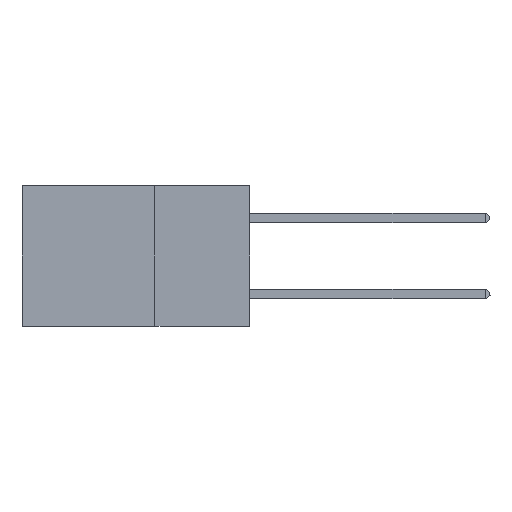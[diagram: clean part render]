
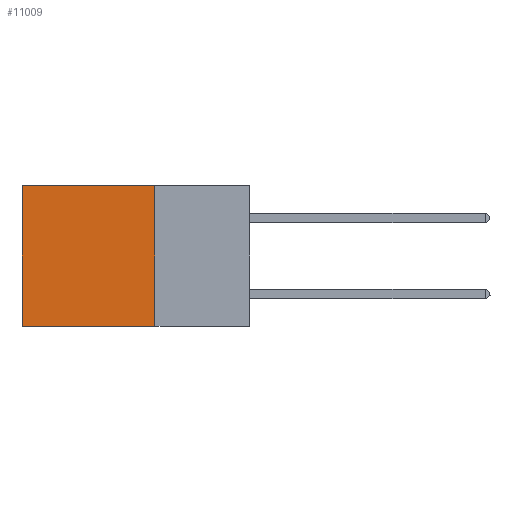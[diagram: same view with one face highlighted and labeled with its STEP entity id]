
A CAD part, left-side view. The second image highlights one B-rep face of the part: STEP entity #11009.
In plain terms, the highlighted planar face has unit normal (-1, 0, 0).
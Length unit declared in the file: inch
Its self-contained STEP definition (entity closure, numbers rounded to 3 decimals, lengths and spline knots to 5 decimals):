
#884 = DIRECTION ( 'NONE',  ( 0., 0., -1. ) ) ;
#1632 = VECTOR ( 'NONE', #884, 39.37008 ) ;
#2352 = CARTESIAN_POINT ( 'NONE',  ( 0.2875, 0.25, 0. ) ) ;
#2392 = ORIENTED_EDGE ( 'NONE', *, *, #11553, .T. ) ;
#2393 = CARTESIAN_POINT ( 'NONE',  ( 0.2875, 0.6, 0. ) ) ;
#2508 = PLANE ( 'NONE',  #12608 ) ;
#3537 = VERTEX_POINT ( 'NONE', #11201 ) ;
#4479 = ORIENTED_EDGE ( 'NONE', *, *, #10463, .F. ) ;
#6075 = EDGE_CURVE ( 'NONE', #9899, #13327, #8644, .T. ) ;
#6918 = DIRECTION ( 'NONE',  ( 0., 1., 0. ) ) ;
#7682 = DIRECTION ( 'NONE',  ( 0., 0., -1. ) ) ;
#7990 = CARTESIAN_POINT ( 'NONE',  ( 0.2875, 0.6, 0. ) ) ;
#8022 = VECTOR ( 'NONE', #6918, 39.37008 ) ;
#8190 = CARTESIAN_POINT ( 'NONE',  ( 0.2875, 0.25, 0. ) ) ;
#8644 = LINE ( 'NONE', #19015, #1632 ) ;
#9435 = LINE ( 'NONE', #2352, #8022 ) ;
#9899 = VERTEX_POINT ( 'NONE', #8190 ) ;
#10092 = DIRECTION ( 'NONE',  ( 0., 0., -1. ) ) ;
#10463 = EDGE_CURVE ( 'NONE', #13327, #3537, #11490, .T. ) ;
#10764 = LINE ( 'NONE', #7990, #15193 ) ;
#11009 = ADVANCED_FACE ( 'NONE', ( #17859 ), #2508, .F. ) ;
#11201 = CARTESIAN_POINT ( 'NONE',  ( 0.2875, 0.6, -0.37 ) ) ;
#11490 = LINE ( 'NONE', #17861, #13829 ) ;
#11553 = EDGE_CURVE ( 'NONE', #9899, #19079, #9435, .T. ) ;
#11558 = EDGE_LOOP ( 'NONE', ( #11972, #4479, #18314, #2392 ) ) ;
#11972 = ORIENTED_EDGE ( 'NONE', *, *, #12540, .T. ) ;
#12540 = EDGE_CURVE ( 'NONE', #19079, #3537, #10764, .T. ) ;
#12608 = AXIS2_PLACEMENT_3D ( 'NONE', #17445, #19008, #10092 ) ;
#13327 = VERTEX_POINT ( 'NONE', #15813 ) ;
#13829 = VECTOR ( 'NONE', #16081, 39.37008 ) ;
#15193 = VECTOR ( 'NONE', #7682, 39.37008 ) ;
#15813 = CARTESIAN_POINT ( 'NONE',  ( 0.2875, 0.25, -0.37 ) ) ;
#16081 = DIRECTION ( 'NONE',  ( 0., 1., 0. ) ) ;
#17445 = CARTESIAN_POINT ( 'NONE',  ( 0.2875, 0.25, 0. ) ) ;
#17859 = FACE_OUTER_BOUND ( 'NONE', #11558, .T. ) ;
#17861 = CARTESIAN_POINT ( 'NONE',  ( 0.2875, 0.25, -0.37 ) ) ;
#18314 = ORIENTED_EDGE ( 'NONE', *, *, #6075, .F. ) ;
#19008 = DIRECTION ( 'NONE',  ( 1., 0., 0. ) ) ;
#19015 = CARTESIAN_POINT ( 'NONE',  ( 0.2875, 0.25, 0. ) ) ;
#19079 = VERTEX_POINT ( 'NONE', #2393 ) ;
